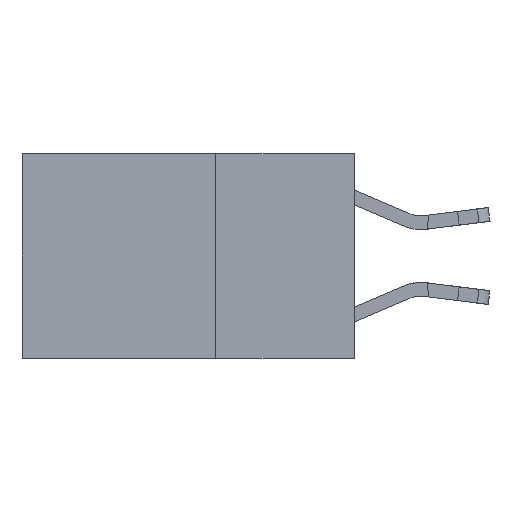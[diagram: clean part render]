
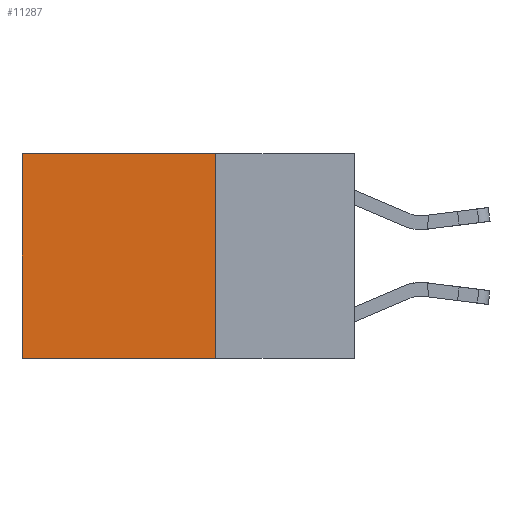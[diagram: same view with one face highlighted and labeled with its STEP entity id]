
A CAD part, left-side view. The second image highlights one B-rep face of the part: STEP entity #11287.
In plain terms, the highlighted planar face has unit normal (-1, 0, 0).
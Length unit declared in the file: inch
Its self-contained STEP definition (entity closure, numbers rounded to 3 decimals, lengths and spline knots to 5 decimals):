
#42 = CARTESIAN_POINT ( 'NONE',  ( 0.2625, 0.6, 0. ) ) ;
#147 = DIRECTION ( 'NONE',  ( 0., 1., 0. ) ) ;
#274 = CARTESIAN_POINT ( 'NONE',  ( 0.2625, 0.25, 0. ) ) ;
#536 = CARTESIAN_POINT ( 'NONE',  ( 0.2625, 0.25, 0. ) ) ;
#637 = LINE ( 'NONE', #19924, #1552 ) ;
#789 = EDGE_CURVE ( 'NONE', #4208, #19263, #11605, .T. ) ;
#905 = ORIENTED_EDGE ( 'NONE', *, *, #6137, .T. ) ;
#1552 = VECTOR ( 'NONE', #18541, 39.37008 ) ;
#2151 = EDGE_CURVE ( 'NONE', #19263, #7786, #637, .T. ) ;
#4208 = VERTEX_POINT ( 'NONE', #536 ) ;
#4708 = AXIS2_PLACEMENT_3D ( 'NONE', #17888, #16223, #14550 ) ;
#5963 = PLANE ( 'NONE',  #4708 ) ;
#6137 = EDGE_CURVE ( 'NONE', #4208, #7343, #16399, .T. ) ;
#7343 = VERTEX_POINT ( 'NONE', #15587 ) ;
#7431 = DIRECTION ( 'NONE',  ( 0., 0., -1. ) ) ;
#7786 = VERTEX_POINT ( 'NONE', #7999 ) ;
#7999 = CARTESIAN_POINT ( 'NONE',  ( 0.2625, 0.6, -0.37 ) ) ;
#8013 = FACE_OUTER_BOUND ( 'NONE', #20060, .T. ) ;
#8176 = LINE ( 'NONE', #42, #15743 ) ;
#9079 = CARTESIAN_POINT ( 'NONE',  ( 0.2625, 0.25, -0.37 ) ) ;
#9481 = ORIENTED_EDGE ( 'NONE', *, *, #9942, .T. ) ;
#9577 = ORIENTED_EDGE ( 'NONE', *, *, #789, .F. ) ;
#9942 = EDGE_CURVE ( 'NONE', #7343, #7786, #8176, .T. ) ;
#11287 = ADVANCED_FACE ( 'NONE', ( #8013 ), #5963, .F. ) ;
#11467 = DIRECTION ( 'NONE',  ( 0., 0., -1. ) ) ;
#11605 = LINE ( 'NONE', #274, #17021 ) ;
#12444 = ORIENTED_EDGE ( 'NONE', *, *, #2151, .F. ) ;
#14550 = DIRECTION ( 'NONE',  ( 0., 0., -1. ) ) ;
#15587 = CARTESIAN_POINT ( 'NONE',  ( 0.2625, 0.6, 0. ) ) ;
#15743 = VECTOR ( 'NONE', #11467, 39.37008 ) ;
#16223 = DIRECTION ( 'NONE',  ( 1., 0., 0. ) ) ;
#16399 = LINE ( 'NONE', #17856, #20897 ) ;
#17021 = VECTOR ( 'NONE', #7431, 39.37008 ) ;
#17856 = CARTESIAN_POINT ( 'NONE',  ( 0.2625, 0.25, 0. ) ) ;
#17888 = CARTESIAN_POINT ( 'NONE',  ( 0.2625, 0.25, 0. ) ) ;
#18541 = DIRECTION ( 'NONE',  ( 0., 1., 0. ) ) ;
#19263 = VERTEX_POINT ( 'NONE', #9079 ) ;
#19924 = CARTESIAN_POINT ( 'NONE',  ( 0.2625, 0.25, -0.37 ) ) ;
#20060 = EDGE_LOOP ( 'NONE', ( #9481, #12444, #9577, #905 ) ) ;
#20897 = VECTOR ( 'NONE', #147, 39.37008 ) ;
